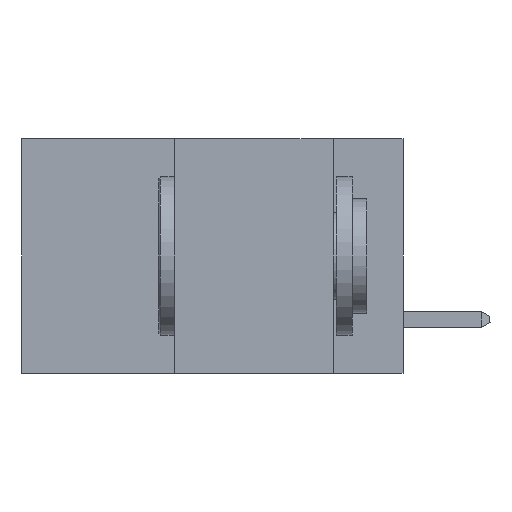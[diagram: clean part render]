
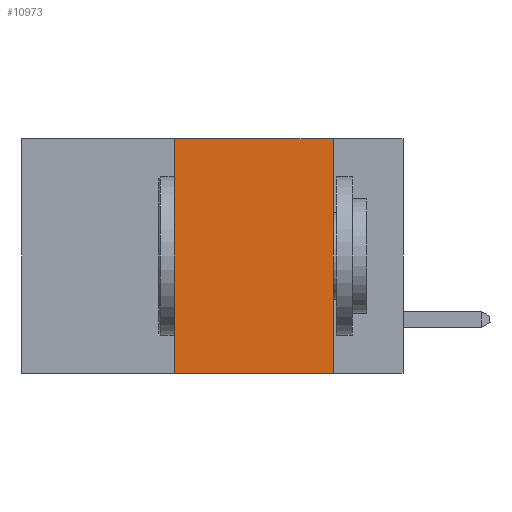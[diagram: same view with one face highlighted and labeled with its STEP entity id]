
A CAD part, left-side view. The second image highlights one B-rep face of the part: STEP entity #10973.
In plain terms, the highlighted planar face has unit normal (-1, 0, 0).
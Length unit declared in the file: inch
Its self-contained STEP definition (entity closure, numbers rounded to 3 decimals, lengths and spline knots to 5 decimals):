
#474 = VECTOR ( 'NONE', #23759, 39.37008 ) ;
#637 = LINE ( 'NONE', #24447, #24799 ) ;
#5876 = ORIENTED_EDGE ( 'NONE', *, *, #16815, .F. ) ;
#8127 = EDGE_CURVE ( 'NONE', #20517, #36160, #21023, .T. ) ;
#9565 = VERTEX_POINT ( 'NONE', #37460 ) ;
#10016 = FACE_OUTER_BOUND ( 'NONE', #21511, .T. ) ;
#10973 = ADVANCED_FACE ( 'NONE', ( #10016 ), #45137, .F. ) ;
#13387 = AXIS2_PLACEMENT_3D ( 'NONE', #15857, #41402, #19618 ) ;
#14160 = CARTESIAN_POINT ( 'NONE',  ( 0., 0.11, 0. ) ) ;
#15129 = ORIENTED_EDGE ( 'NONE', *, *, #21041, .F. ) ;
#15416 = LINE ( 'NONE', #17741, #16004 ) ;
#15857 = CARTESIAN_POINT ( 'NONE',  ( 0., 0.6, 0. ) ) ;
#16004 = VECTOR ( 'NONE', #33110, 39.37008 ) ;
#16815 = EDGE_CURVE ( 'NONE', #9565, #40536, #637, .T. ) ;
#17741 = CARTESIAN_POINT ( 'NONE',  ( 0., 0.6, 0. ) ) ;
#19337 = VECTOR ( 'NONE', #28451, 39.37008 ) ;
#19618 = DIRECTION ( 'NONE',  ( 0., 0., -1. ) ) ;
#20517 = VERTEX_POINT ( 'NONE', #23170 ) ;
#21023 = LINE ( 'NONE', #14160, #19337 ) ;
#21041 = EDGE_CURVE ( 'NONE', #40536, #20517, #15416, .T. ) ;
#21511 = EDGE_LOOP ( 'NONE', ( #44319, #15129, #5876, #44488 ) ) ;
#22971 = LINE ( 'NONE', #34530, #474 ) ;
#23170 = CARTESIAN_POINT ( 'NONE',  ( 0., 0.11, 0. ) ) ;
#23759 = DIRECTION ( 'NONE',  ( 0., -1., 0. ) ) ;
#24447 = CARTESIAN_POINT ( 'NONE',  ( 0., 0.36, 0. ) ) ;
#24799 = VECTOR ( 'NONE', #37401, 39.37008 ) ;
#28045 = EDGE_CURVE ( 'NONE', #9565, #36160, #22971, .T. ) ;
#28451 = DIRECTION ( 'NONE',  ( 0., 0., -1. ) ) ;
#32730 = CARTESIAN_POINT ( 'NONE',  ( 0., 0.11, -0.37 ) ) ;
#33110 = DIRECTION ( 'NONE',  ( 0., -1., 0. ) ) ;
#34530 = CARTESIAN_POINT ( 'NONE',  ( 0., 0.6, -0.37 ) ) ;
#34743 = CARTESIAN_POINT ( 'NONE',  ( 0., 0.36, 0. ) ) ;
#36160 = VERTEX_POINT ( 'NONE', #32730 ) ;
#37401 = DIRECTION ( 'NONE',  ( 0., 0., 1. ) ) ;
#37460 = CARTESIAN_POINT ( 'NONE',  ( 0., 0.36, -0.37 ) ) ;
#40536 = VERTEX_POINT ( 'NONE', #34743 ) ;
#41402 = DIRECTION ( 'NONE',  ( 1., 0., 0. ) ) ;
#44319 = ORIENTED_EDGE ( 'NONE', *, *, #8127, .F. ) ;
#44488 = ORIENTED_EDGE ( 'NONE', *, *, #28045, .T. ) ;
#45137 = PLANE ( 'NONE',  #13387 ) ;
